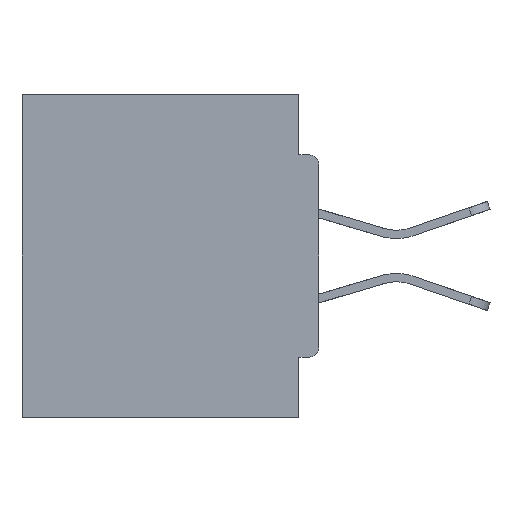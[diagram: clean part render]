
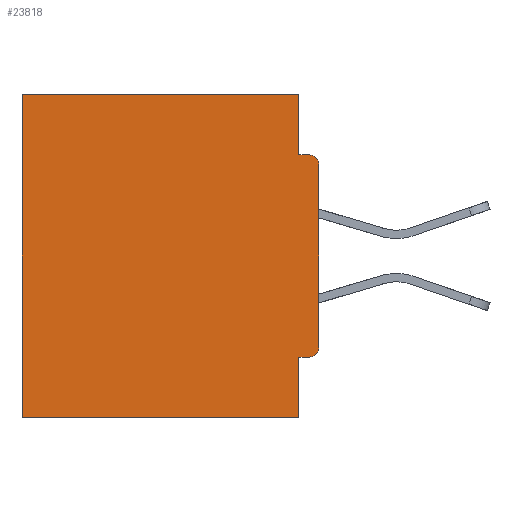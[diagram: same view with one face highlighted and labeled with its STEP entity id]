
A CAD part, left-side view. The second image highlights one B-rep face of the part: STEP entity #23818.
In plain terms, the highlighted planar face has unit normal (-1, 0, 0).
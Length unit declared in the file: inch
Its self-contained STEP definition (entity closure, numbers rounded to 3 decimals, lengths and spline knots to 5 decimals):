
#129 = CARTESIAN_POINT ( 'NONE',  ( 0.298, 0.031, -0.5 ) ) ;
#747 = CARTESIAN_POINT ( 'NONE',  ( 0.298, 0., 0. ) ) ;
#794 = VERTEX_POINT ( 'NONE', #31697 ) ;
#1471 = LINE ( 'NONE', #29375, #19879 ) ;
#1966 = CARTESIAN_POINT ( 'NONE',  ( 0.298, 0.031, 0. ) ) ;
#1967 = EDGE_CURVE ( 'NONE', #31480, #11570, #28567, .T. ) ;
#2546 = DIRECTION ( 'NONE',  ( 0., 0., -1. ) ) ;
#2976 = VECTOR ( 'NONE', #12507, 39.37008 ) ;
#3054 = VERTEX_POINT ( 'NONE', #1966 ) ;
#3206 = EDGE_CURVE ( 'NONE', #20663, #22957, #24620, .T. ) ;
#3234 = DIRECTION ( 'NONE',  ( 0., 1., 0. ) ) ;
#3372 = AXIS2_PLACEMENT_3D ( 'NONE', #17947, #25103, #10106 ) ;
#3420 = VERTEX_POINT ( 'NONE', #9021 ) ;
#3802 = ORIENTED_EDGE ( 'NONE', *, *, #23268, .F. ) ;
#3939 = CARTESIAN_POINT ( 'NONE',  ( 0.298, 0.015, -0.4065 ) ) ;
#4174 = CARTESIAN_POINT ( 'NONE',  ( 0.298, 0.031, -0.5 ) ) ;
#4350 = CARTESIAN_POINT ( 'NONE',  ( 0.298, 0.031, -0.5 ) ) ;
#4489 = CARTESIAN_POINT ( 'NONE',  ( 0.298, 0.031, -0.0935 ) ) ;
#5008 = ORIENTED_EDGE ( 'NONE', *, *, #1967, .F. ) ;
#5017 = CARTESIAN_POINT ( 'NONE',  ( 0.298, 0., -0.4065 ) ) ;
#5684 = AXIS2_PLACEMENT_3D ( 'NONE', #30006, #25426, #2546 ) ;
#5727 = ORIENTED_EDGE ( 'NONE', *, *, #7143, .F. ) ;
#7143 = EDGE_CURVE ( 'NONE', #3054, #23303, #19960, .T. ) ;
#7372 = VECTOR ( 'NONE', #7709, 39.37008 ) ;
#7709 = DIRECTION ( 'NONE',  ( 0., 0., -1. ) ) ;
#8756 = ORIENTED_EDGE ( 'NONE', *, *, #19114, .F. ) ;
#9021 = CARTESIAN_POINT ( 'NONE',  ( 0.298, 0.46, -0.5 ) ) ;
#9405 = EDGE_CURVE ( 'NONE', #794, #3420, #10346, .T. ) ;
#9904 = DIRECTION ( 'NONE',  ( 1., 0., 0. ) ) ;
#10015 = DIRECTION ( 'NONE',  ( 0., 1., 0. ) ) ;
#10090 = CARTESIAN_POINT ( 'NONE',  ( 0.298, 0.46, 0. ) ) ;
#10106 = DIRECTION ( 'NONE',  ( 0., 0., -1. ) ) ;
#10108 = DIRECTION ( 'NONE',  ( 0., 0., -1. ) ) ;
#10346 = LINE ( 'NONE', #10090, #2976 ) ;
#10388 = LINE ( 'NONE', #747, #22994 ) ;
#11570 = VERTEX_POINT ( 'NONE', #4350 ) ;
#11874 = PLANE ( 'NONE',  #28016 ) ;
#12507 = DIRECTION ( 'NONE',  ( 0., 0., -1. ) ) ;
#13376 = VECTOR ( 'NONE', #17960, 39.37008 ) ;
#14667 = ORIENTED_EDGE ( 'NONE', *, *, #25614, .F. ) ;
#14852 = VECTOR ( 'NONE', #25865, 39.37008 ) ;
#16272 = FACE_OUTER_BOUND ( 'NONE', #25192, .T. ) ;
#16314 = VERTEX_POINT ( 'NONE', #25442 ) ;
#16328 = EDGE_CURVE ( 'NONE', #20663, #16314, #21545, .T. ) ;
#17465 = LINE ( 'NONE', #5017, #31914 ) ;
#17745 = CARTESIAN_POINT ( 'NONE',  ( 0.298, 0., -0.0935 ) ) ;
#17763 = EDGE_CURVE ( 'NONE', #3054, #794, #10388, .T. ) ;
#17947 = CARTESIAN_POINT ( 'NONE',  ( 0.298, 0.015, -0.3915 ) ) ;
#17960 = DIRECTION ( 'NONE',  ( 0., -1., 0. ) ) ;
#18274 = VERTEX_POINT ( 'NONE', #3939 ) ;
#18303 = CARTESIAN_POINT ( 'NONE',  ( 0.298, 0., 0. ) ) ;
#19112 = CARTESIAN_POINT ( 'NONE',  ( 0.298, 0., -0.1085 ) ) ;
#19114 = EDGE_CURVE ( 'NONE', #23303, #22957, #31045, .T. ) ;
#19238 = CIRCLE ( 'NONE', #3372, 0.015 ) ;
#19243 = ORIENTED_EDGE ( 'NONE', *, *, #17763, .T. ) ;
#19879 = VECTOR ( 'NONE', #29488, 39.37008 ) ;
#19960 = LINE ( 'NONE', #4174, #27753 ) ;
#20663 = VERTEX_POINT ( 'NONE', #19112 ) ;
#21545 = LINE ( 'NONE', #18303, #14852 ) ;
#21732 = ORIENTED_EDGE ( 'NONE', *, *, #9405, .T. ) ;
#21852 = ORIENTED_EDGE ( 'NONE', *, *, #3206, .T. ) ;
#22957 = VERTEX_POINT ( 'NONE', #28010 ) ;
#22994 = VECTOR ( 'NONE', #3234, 39.37008 ) ;
#23268 = EDGE_CURVE ( 'NONE', #11570, #3420, #1471, .T. ) ;
#23303 = VERTEX_POINT ( 'NONE', #4489 ) ;
#23722 = DIRECTION ( 'NONE',  ( 0., 0., -1. ) ) ;
#23818 = ADVANCED_FACE ( 'NONE', ( #16272 ), #11874, .F. ) ;
#23954 = CARTESIAN_POINT ( 'NONE',  ( 0.298, 0.031, -0.4065 ) ) ;
#24620 = CIRCLE ( 'NONE', #5684, 0.015 ) ;
#25103 = DIRECTION ( 'NONE',  ( -1., 0., 0. ) ) ;
#25192 = EDGE_LOOP ( 'NONE', ( #21852, #8756, #5727, #19243, #21732, #3802, #5008, #14667, #31919, #25395 ) ) ;
#25204 = CARTESIAN_POINT ( 'NONE',  ( 0.298, 0., 0. ) ) ;
#25395 = ORIENTED_EDGE ( 'NONE', *, *, #16328, .F. ) ;
#25426 = DIRECTION ( 'NONE',  ( -1., 0., 0. ) ) ;
#25442 = CARTESIAN_POINT ( 'NONE',  ( 0.298, 0., -0.3915 ) ) ;
#25614 = EDGE_CURVE ( 'NONE', #18274, #31480, #17465, .T. ) ;
#25865 = DIRECTION ( 'NONE',  ( 0., 0., -1. ) ) ;
#27753 = VECTOR ( 'NONE', #23722, 39.37008 ) ;
#28010 = CARTESIAN_POINT ( 'NONE',  ( 0.298, 0.015, -0.0935 ) ) ;
#28016 = AXIS2_PLACEMENT_3D ( 'NONE', #25204, #9904, #10108 ) ;
#28384 = EDGE_CURVE ( 'NONE', #18274, #16314, #19238, .T. ) ;
#28567 = LINE ( 'NONE', #129, #7372 ) ;
#29375 = CARTESIAN_POINT ( 'NONE',  ( 0.298, 0., -0.5 ) ) ;
#29488 = DIRECTION ( 'NONE',  ( 0., 1., 0. ) ) ;
#30006 = CARTESIAN_POINT ( 'NONE',  ( 0.298, 0.015, -0.1085 ) ) ;
#31045 = LINE ( 'NONE', #17745, #13376 ) ;
#31480 = VERTEX_POINT ( 'NONE', #23954 ) ;
#31697 = CARTESIAN_POINT ( 'NONE',  ( 0.298, 0.46, 0. ) ) ;
#31914 = VECTOR ( 'NONE', #10015, 39.37008 ) ;
#31919 = ORIENTED_EDGE ( 'NONE', *, *, #28384, .T. ) ;
